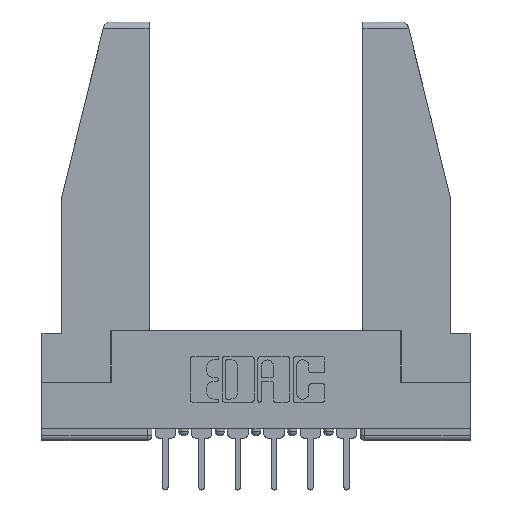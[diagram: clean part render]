
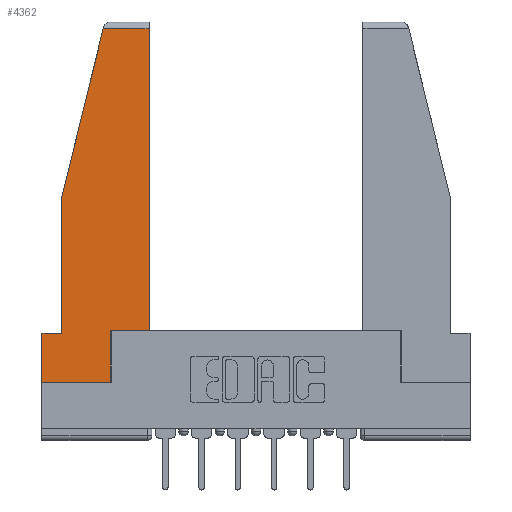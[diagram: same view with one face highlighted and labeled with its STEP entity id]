
A CAD part, top view. The second image highlights one B-rep face of the part: STEP entity #4362.
In plain terms, the highlighted planar face has unit normal (0, 0, 1).
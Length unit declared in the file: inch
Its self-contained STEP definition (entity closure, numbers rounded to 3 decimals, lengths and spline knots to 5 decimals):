
#17 = VECTOR ( 'NONE', #9147, 39.37008 ) ;
#21 = VERTEX_POINT ( 'NONE', #10577 ) ;
#178 = FACE_OUTER_BOUND ( 'NONE', #5267, .T. ) ;
#213 = CARTESIAN_POINT ( 'NONE',  ( 0.461, 0.223, 0. ) ) ;
#237 = LINE ( 'NONE', #9663, #1989 ) ;
#257 = CARTESIAN_POINT ( 'NONE',  ( 0.086, 0.21, 0. ) ) ;
#371 = EDGE_CURVE ( 'NONE', #10370, #8226, #10581, .T. ) ;
#394 = AXIS2_PLACEMENT_3D ( 'NONE', #9493, #1062, #1178 ) ;
#446 = EDGE_CURVE ( 'NONE', #10235, #2450, #7634, .T. ) ;
#650 = CARTESIAN_POINT ( 'NONE',  ( 0.297, 0.223, 0. ) ) ;
#970 = DIRECTION ( 'NONE',  ( 0., 1., 0. ) ) ;
#992 = VECTOR ( 'NONE', #2082, 39.37008 ) ;
#1059 = CARTESIAN_POINT ( 'NONE',  ( 0., 0.21, 0. ) ) ;
#1062 = DIRECTION ( 'NONE',  ( 0., 0., 1. ) ) ;
#1148 = LINE ( 'NONE', #1951, #992 ) ;
#1178 = DIRECTION ( 'NONE',  ( 1., 0., 0. ) ) ;
#1302 = CARTESIAN_POINT ( 'NONE',  ( 0.271, 1.55, 0. ) ) ;
#1436 = VERTEX_POINT ( 'NONE', #257 ) ;
#1638 = LINE ( 'NONE', #10138, #17 ) ;
#1790 = ORIENTED_EDGE ( 'NONE', *, *, #5217, .T. ) ;
#1951 = CARTESIAN_POINT ( 'NONE',  ( 0., 0., 0. ) ) ;
#1989 = VECTOR ( 'NONE', #2954, 39.37008 ) ;
#2026 = LINE ( 'NONE', #7563, #9665 ) ;
#2082 = DIRECTION ( 'NONE',  ( 1., 0., 0. ) ) ;
#2118 = EDGE_CURVE ( 'NONE', #2450, #10185, #1148, .T. ) ;
#2211 = ORIENTED_EDGE ( 'NONE', *, *, #10249, .T. ) ;
#2217 = VERTEX_POINT ( 'NONE', #213 ) ;
#2282 = EDGE_CURVE ( 'NONE', #8305, #2217, #11681, .T. ) ;
#2450 = VERTEX_POINT ( 'NONE', #10248 ) ;
#2458 = VECTOR ( 'NONE', #11339, 39.37008 ) ;
#2891 = DIRECTION ( 'NONE',  ( -1., 0., 0. ) ) ;
#2954 = DIRECTION ( 'NONE',  ( 0., 1., 0. ) ) ;
#3738 = CARTESIAN_POINT ( 'NONE',  ( 0.297, 0., 0. ) ) ;
#4146 = ORIENTED_EDGE ( 'NONE', *, *, #446, .T. ) ;
#4362 = ADVANCED_FACE ( 'NONE', ( #178 ), #9606, .T. ) ;
#4574 = ORIENTED_EDGE ( 'NONE', *, *, #2282, .T. ) ;
#4804 = DIRECTION ( 'NONE',  ( 0., -1., 0. ) ) ;
#4818 = EDGE_CURVE ( 'NONE', #1436, #10235, #6630, .T. ) ;
#5033 = DIRECTION ( 'NONE',  ( -0.239, -0.971, 0. ) ) ;
#5217 = EDGE_CURVE ( 'NONE', #21, #10370, #1638, .T. ) ;
#5267 = EDGE_LOOP ( 'NONE', ( #2211, #1790, #8940, #5939, #10754, #4146, #9217, #7950, #4574 ) ) ;
#5939 = ORIENTED_EDGE ( 'NONE', *, *, #8884, .T. ) ;
#6304 = CARTESIAN_POINT ( 'NONE',  ( 0.086, 0.8, 0. ) ) ;
#6630 = LINE ( 'NONE', #9536, #12024 ) ;
#6740 = CARTESIAN_POINT ( 'NONE',  ( 0., 0.21, 0. ) ) ;
#6973 = CARTESIAN_POINT ( 'NONE',  ( 0.297, 0.223, 0. ) ) ;
#7563 = CARTESIAN_POINT ( 'NONE',  ( 0.461, 0.223, 0. ) ) ;
#7634 = LINE ( 'NONE', #1059, #9212 ) ;
#7950 = ORIENTED_EDGE ( 'NONE', *, *, #9802, .T. ) ;
#8226 = VERTEX_POINT ( 'NONE', #6304 ) ;
#8305 = VERTEX_POINT ( 'NONE', #650 ) ;
#8469 = VECTOR ( 'NONE', #10737, 39.37008 ) ;
#8504 = LINE ( 'NONE', #8563, #2458 ) ;
#8563 = CARTESIAN_POINT ( 'NONE',  ( 0.086, 0.8, 0. ) ) ;
#8884 = EDGE_CURVE ( 'NONE', #8226, #1436, #8504, .T. ) ;
#8940 = ORIENTED_EDGE ( 'NONE', *, *, #371, .T. ) ;
#8974 = CARTESIAN_POINT ( 'NONE',  ( 0.2636, 1.52, 0. ) ) ;
#9147 = DIRECTION ( 'NONE',  ( -1., 0., 0. ) ) ;
#9212 = VECTOR ( 'NONE', #4804, 39.37008 ) ;
#9217 = ORIENTED_EDGE ( 'NONE', *, *, #2118, .T. ) ;
#9493 = CARTESIAN_POINT ( 'NONE',  ( 0., 0., 0. ) ) ;
#9536 = CARTESIAN_POINT ( 'NONE',  ( 0., 0.21, 0. ) ) ;
#9606 = PLANE ( 'NONE',  #394 ) ;
#9663 = CARTESIAN_POINT ( 'NONE',  ( 0.297, 0., 0. ) ) ;
#9665 = VECTOR ( 'NONE', #970, 39.37008 ) ;
#9802 = EDGE_CURVE ( 'NONE', #10185, #8305, #237, .T. ) ;
#10138 = CARTESIAN_POINT ( 'NONE',  ( 0., 1.52, 0. ) ) ;
#10185 = VERTEX_POINT ( 'NONE', #3738 ) ;
#10235 = VERTEX_POINT ( 'NONE', #6740 ) ;
#10248 = CARTESIAN_POINT ( 'NONE',  ( 0., 0., 0. ) ) ;
#10249 = EDGE_CURVE ( 'NONE', #2217, #21, #2026, .T. ) ;
#10370 = VERTEX_POINT ( 'NONE', #8974 ) ;
#10577 = CARTESIAN_POINT ( 'NONE',  ( 0.461, 1.52, 0. ) ) ;
#10581 = LINE ( 'NONE', #1302, #11773 ) ;
#10737 = DIRECTION ( 'NONE',  ( 1., 0., 0. ) ) ;
#10754 = ORIENTED_EDGE ( 'NONE', *, *, #4818, .T. ) ;
#11339 = DIRECTION ( 'NONE',  ( 0., -1., 0. ) ) ;
#11681 = LINE ( 'NONE', #6973, #8469 ) ;
#11773 = VECTOR ( 'NONE', #5033, 39.37008 ) ;
#12024 = VECTOR ( 'NONE', #2891, 39.37008 ) ;
